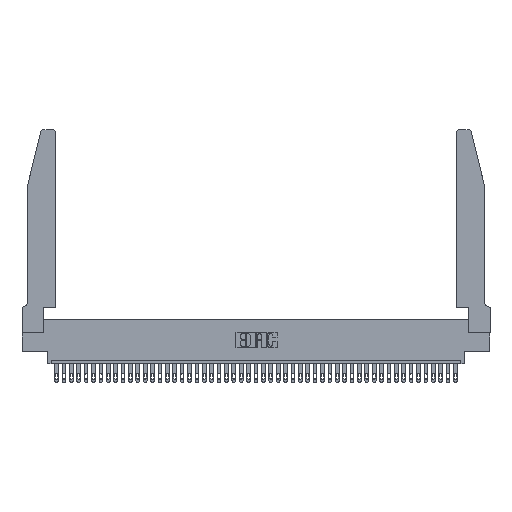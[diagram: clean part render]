
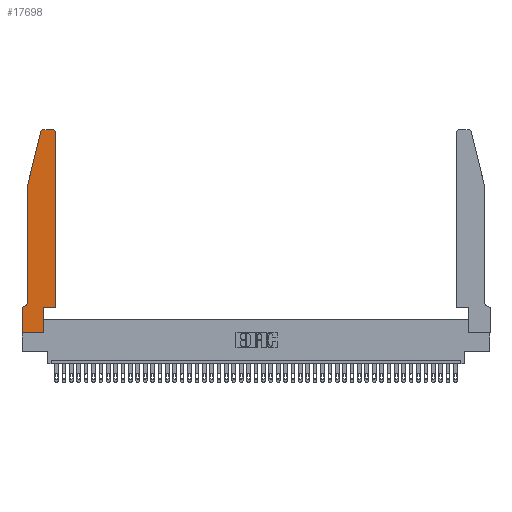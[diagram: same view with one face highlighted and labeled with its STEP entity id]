
A CAD part, top view. The second image highlights one B-rep face of the part: STEP entity #17698.
In plain terms, the highlighted planar face has unit normal (0, 0, 1).
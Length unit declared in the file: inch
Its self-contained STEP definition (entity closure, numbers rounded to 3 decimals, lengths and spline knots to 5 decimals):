
#114 = ORIENTED_EDGE ( 'NONE', *, *, #27056, .T. ) ;
#749 = CARTESIAN_POINT ( 'NONE',  ( 0.4505, 0.35, 0.37 ) ) ;
#2245 = CARTESIAN_POINT ( 'NONE',  ( 0.2865, 0., 0.37 ) ) ;
#2467 = DIRECTION ( 'NONE',  ( 1., 0., 0. ) ) ;
#2733 = CARTESIAN_POINT ( 'NONE',  ( 0., 0., 0.37 ) ) ;
#3955 = DIRECTION ( 'NONE',  ( 0., 1., 0. ) ) ;
#5267 = LINE ( 'NONE', #14698, #42297 ) ;
#6107 = EDGE_CURVE ( 'NONE', #26377, #18416, #9271, .T. ) ;
#6208 = ORIENTED_EDGE ( 'NONE', *, *, #6107, .T. ) ;
#6551 = ORIENTED_EDGE ( 'NONE', *, *, #34701, .T. ) ;
#6842 = LINE ( 'NONE', #44181, #27715 ) ;
#6981 = DIRECTION ( 'NONE',  ( 0., -1., 0. ) ) ;
#7405 = CARTESIAN_POINT ( 'NONE',  ( 0.4505, 2.72, 0.37 ) ) ;
#7557 = DIRECTION ( 'NONE',  ( 1., 0., 0. ) ) ;
#7571 = CARTESIAN_POINT ( 'NONE',  ( 0.2865, 0.35, 0.37 ) ) ;
#7581 = EDGE_CURVE ( 'NONE', #33451, #10037, #10430, .T. ) ;
#7588 = VERTEX_POINT ( 'NONE', #7405 ) ;
#8196 = CARTESIAN_POINT ( 'NONE',  ( 0.25487, 2.72718, 0.37 ) ) ;
#9271 = LINE ( 'NONE', #11696, #35521 ) ;
#9569 = VERTEX_POINT ( 'NONE', #8196 ) ;
#9709 = ORIENTED_EDGE ( 'NONE', *, *, #20625, .T. ) ;
#9987 = DIRECTION ( 'NONE',  ( -1., 0., 0. ) ) ;
#10037 = VERTEX_POINT ( 'NONE', #2245 ) ;
#10156 = DIRECTION ( 'NONE',  ( 0., 0., 1. ) ) ;
#10209 = VERTEX_POINT ( 'NONE', #14475 ) ;
#10430 = LINE ( 'NONE', #34281, #37785 ) ;
#10784 = CARTESIAN_POINT ( 'NONE',  ( 0.284, 2.75, 0.37 ) ) ;
#11696 = CARTESIAN_POINT ( 'NONE',  ( 0.0755, 2., 0.37 ) ) ;
#12056 = ORIENTED_EDGE ( 'NONE', *, *, #19574, .T. ) ;
#13125 = ORIENTED_EDGE ( 'NONE', *, *, #25515, .T. ) ;
#13143 = AXIS2_PLACEMENT_3D ( 'NONE', #20430, #10156, #17282 ) ;
#14475 = CARTESIAN_POINT ( 'NONE',  ( 0.4205, 2.75, 0.37 ) ) ;
#14698 = CARTESIAN_POINT ( 'NONE',  ( 0.0755, 2., 0.37 ) ) ;
#14723 = PLANE ( 'NONE',  #15908 ) ;
#14889 = CARTESIAN_POINT ( 'NONE',  ( 0.4505, 0.35, 0.37 ) ) ;
#14991 = LINE ( 'NONE', #749, #23620 ) ;
#15323 = CARTESIAN_POINT ( 'NONE',  ( 0.0055, 0.42, 0.37 ) ) ;
#15908 = AXIS2_PLACEMENT_3D ( 'NONE', #42194, #18153, #7557 ) ;
#16310 = CIRCLE ( 'NONE', #33917, 0.07 ) ;
#17165 = DIRECTION ( 'NONE',  ( 1., 0., 0. ) ) ;
#17183 = ORIENTED_EDGE ( 'NONE', *, *, #30718, .T. ) ;
#17282 = DIRECTION ( 'NONE',  ( 1., 0., 0. ) ) ;
#17698 = ADVANCED_FACE ( 'NONE', ( #42628 ), #14723, .T. ) ;
#18153 = DIRECTION ( 'NONE',  ( 0., 0., 1. ) ) ;
#18416 = VERTEX_POINT ( 'NONE', #38282 ) ;
#19130 = DIRECTION ( 'NONE',  ( 1., 0., 0. ) ) ;
#19574 = EDGE_CURVE ( 'NONE', #43963, #43973, #31683, .T. ) ;
#19835 = ORIENTED_EDGE ( 'NONE', *, *, #37493, .T. ) ;
#20430 = CARTESIAN_POINT ( 'NONE',  ( 0.4205, 2.72, 0.37 ) ) ;
#20441 = DIRECTION ( 'NONE',  ( -1., 0., 0. ) ) ;
#20546 = VECTOR ( 'NONE', #9987, 39.37008 ) ;
#20625 = EDGE_CURVE ( 'NONE', #7588, #10209, #39422, .T. ) ;
#21151 = CARTESIAN_POINT ( 'NONE',  ( 0.2865, 0.35, 0.37 ) ) ;
#21325 = CARTESIAN_POINT ( 'NONE',  ( 0.0755, 2., 0.37 ) ) ;
#21597 = DIRECTION ( 'NONE',  ( -1., 0., 0. ) ) ;
#22062 = EDGE_CURVE ( 'NONE', #10037, #43963, #28485, .T. ) ;
#22585 = AXIS2_PLACEMENT_3D ( 'NONE', #29655, #23035, #19130 ) ;
#23035 = DIRECTION ( 'NONE',  ( 0., 0., 1. ) ) ;
#23620 = VECTOR ( 'NONE', #3955, 39.37008 ) ;
#24703 = VECTOR ( 'NONE', #2467, 39.37008 ) ;
#25515 = EDGE_CURVE ( 'NONE', #10209, #43235, #6842, .T. ) ;
#26377 = VERTEX_POINT ( 'NONE', #21325 ) ;
#27056 = EDGE_CURVE ( 'NONE', #43973, #7588, #14991, .T. ) ;
#27106 = LINE ( 'NONE', #34135, #44258 ) ;
#27394 = CIRCLE ( 'NONE', #22585, 0.03 ) ;
#27715 = VECTOR ( 'NONE', #20441, 39.37008 ) ;
#27847 = VERTEX_POINT ( 'NONE', #31510 ) ;
#27938 = DIRECTION ( 'NONE',  ( 0., 1., 0. ) ) ;
#28206 = DIRECTION ( 'NONE',  ( -0.239, -0.971, 0. ) ) ;
#28485 = LINE ( 'NONE', #21151, #29015 ) ;
#28974 = ORIENTED_EDGE ( 'NONE', *, *, #22062, .T. ) ;
#29015 = VECTOR ( 'NONE', #27938, 39.37008 ) ;
#29655 = CARTESIAN_POINT ( 'NONE',  ( 0.284, 2.72, 0.37 ) ) ;
#30368 = CARTESIAN_POINT ( 'NONE',  ( 0.0755, 0.35, 0.37 ) ) ;
#30718 = EDGE_CURVE ( 'NONE', #42623, #33451, #27106, .T. ) ;
#31510 = CARTESIAN_POINT ( 'NONE',  ( 0.0055, 0.35, 0.37 ) ) ;
#31683 = LINE ( 'NONE', #36032, #24703 ) ;
#31910 = ORIENTED_EDGE ( 'NONE', *, *, #36410, .T. ) ;
#32173 = ORIENTED_EDGE ( 'NONE', *, *, #34443, .T. ) ;
#32589 = DIRECTION ( 'NONE',  ( 0., 0., -1. ) ) ;
#33451 = VERTEX_POINT ( 'NONE', #2733 ) ;
#33917 = AXIS2_PLACEMENT_3D ( 'NONE', #15323, #32589, #21597 ) ;
#34135 = CARTESIAN_POINT ( 'NONE',  ( 0., 0., 0.37 ) ) ;
#34281 = CARTESIAN_POINT ( 'NONE',  ( 0., 0., 0.37 ) ) ;
#34443 = EDGE_CURVE ( 'NONE', #18416, #27847, #16310, .T. ) ;
#34701 = EDGE_CURVE ( 'NONE', #27847, #42623, #41487, .T. ) ;
#35521 = VECTOR ( 'NONE', #35699, 39.37008 ) ;
#35699 = DIRECTION ( 'NONE',  ( 0., -1., 0. ) ) ;
#35804 = EDGE_LOOP ( 'NONE', ( #13125, #31910, #19835, #6208, #32173, #6551, #17183, #39947, #28974, #12056, #114, #9709 ) ) ;
#36032 = CARTESIAN_POINT ( 'NONE',  ( 0.4505, 0.35, 0.37 ) ) ;
#36410 = EDGE_CURVE ( 'NONE', #43235, #9569, #27394, .T. ) ;
#37493 = EDGE_CURVE ( 'NONE', #9569, #26377, #5267, .T. ) ;
#37785 = VECTOR ( 'NONE', #17165, 39.37008 ) ;
#38282 = CARTESIAN_POINT ( 'NONE',  ( 0.0755, 0.42, 0.37 ) ) ;
#38865 = CARTESIAN_POINT ( 'NONE',  ( 0., 0.35, 0.37 ) ) ;
#39422 = CIRCLE ( 'NONE', #13143, 0.03 ) ;
#39947 = ORIENTED_EDGE ( 'NONE', *, *, #7581, .T. ) ;
#41487 = LINE ( 'NONE', #30368, #20546 ) ;
#42194 = CARTESIAN_POINT ( 'NONE',  ( 0., 0.35, 0.37 ) ) ;
#42297 = VECTOR ( 'NONE', #28206, 39.37008 ) ;
#42623 = VERTEX_POINT ( 'NONE', #38865 ) ;
#42628 = FACE_OUTER_BOUND ( 'NONE', #35804, .T. ) ;
#43235 = VERTEX_POINT ( 'NONE', #10784 ) ;
#43963 = VERTEX_POINT ( 'NONE', #7571 ) ;
#43973 = VERTEX_POINT ( 'NONE', #14889 ) ;
#44181 = CARTESIAN_POINT ( 'NONE',  ( 0.2605, 2.75, 0.37 ) ) ;
#44258 = VECTOR ( 'NONE', #6981, 39.37008 ) ;
